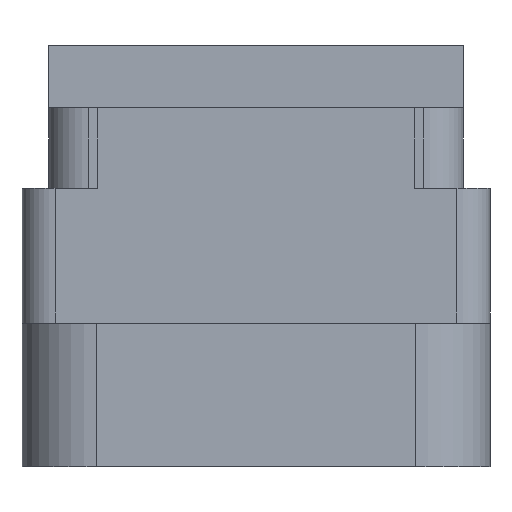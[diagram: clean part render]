
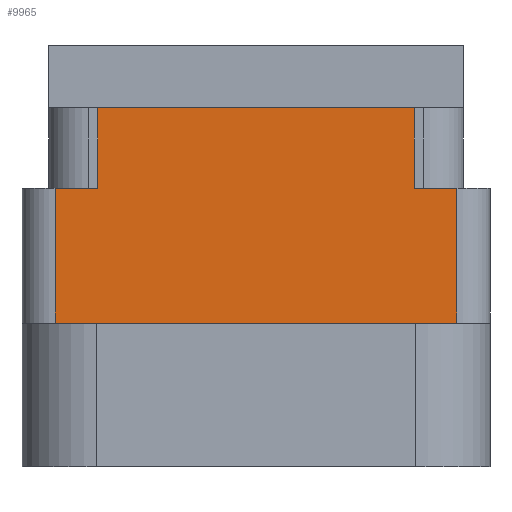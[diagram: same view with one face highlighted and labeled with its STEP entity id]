
A CAD part, left-side view. The second image highlights one B-rep face of the part: STEP entity #9965.
In plain terms, the highlighted planar face has unit normal (-1, 0, 0).
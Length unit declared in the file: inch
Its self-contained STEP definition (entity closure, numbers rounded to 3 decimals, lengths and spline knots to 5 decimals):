
#781 = ORIENTED_EDGE ( 'NONE', *, *, #7627, .F. ) ;
#800 = DIRECTION ( 'NONE',  ( 0., 0., -1. ) ) ;
#829 = CARTESIAN_POINT ( 'NONE',  ( -1., 0., -0.52 ) ) ;
#1359 = CARTESIAN_POINT ( 'NONE',  ( -1., 0.438, -0.117 ) ) ;
#2699 = ORIENTED_EDGE ( 'NONE', *, *, #14795, .T. ) ;
#3583 = LINE ( 'NONE', #25092, #16459 ) ;
#4139 = PLANE ( 'NONE',  #21586 ) ;
#4906 = LINE ( 'NONE', #26432, #11328 ) ;
#5206 = CARTESIAN_POINT ( 'NONE',  ( -1., -0.296, -0.268 ) ) ;
#5990 = ORIENTED_EDGE ( 'NONE', *, *, #13882, .F. ) ;
#6275 = VECTOR ( 'NONE', #800, 39.37008 ) ;
#7132 = VECTOR ( 'NONE', #29669, 39.37008 ) ;
#7178 = VERTEX_POINT ( 'NONE', #7757 ) ;
#7310 = CARTESIAN_POINT ( 'NONE',  ( -1., 0.376, -0.789 ) ) ;
#7619 = CARTESIAN_POINT ( 'NONE',  ( -1., 0.296, -0.268 ) ) ;
#7627 = EDGE_CURVE ( 'NONE', #20608, #7178, #20524, .T. ) ;
#7757 = CARTESIAN_POINT ( 'NONE',  ( -1., 0.296, -0.117 ) ) ;
#8658 = CARTESIAN_POINT ( 'NONE',  ( -1., -0.438, -0.789 ) ) ;
#8697 = CARTESIAN_POINT ( 'NONE',  ( -1., 0.376, -0.268 ) ) ;
#9180 = CARTESIAN_POINT ( 'NONE',  ( -1., -0.376, -0.789 ) ) ;
#9965 = ADVANCED_FACE ( 'NONE', ( #15332 ), #4139, .T. ) ;
#10015 = DIRECTION ( 'NONE',  ( 0., 0., 1. ) ) ;
#10758 = ORIENTED_EDGE ( 'NONE', *, *, #21530, .T. ) ;
#11161 = LINE ( 'NONE', #829, #17992 ) ;
#11328 = VECTOR ( 'NONE', #20034, 39.37008 ) ;
#12060 = EDGE_LOOP ( 'NONE', ( #5990, #2699, #23293, #23533, #17373, #10758, #25731, #781 ) ) ;
#12412 = VERTEX_POINT ( 'NONE', #27293 ) ;
#13398 = EDGE_CURVE ( 'NONE', #14113, #15304, #16719, .T. ) ;
#13882 = EDGE_CURVE ( 'NONE', #17393, #20608, #4906, .T. ) ;
#14113 = VERTEX_POINT ( 'NONE', #5206 ) ;
#14179 = CARTESIAN_POINT ( 'NONE',  ( -1., -0.376, -0.268 ) ) ;
#14795 = EDGE_CURVE ( 'NONE', #17393, #21292, #26772, .T. ) ;
#15304 = VERTEX_POINT ( 'NONE', #14179 ) ;
#15332 = FACE_OUTER_BOUND ( 'NONE', #12060, .T. ) ;
#15593 = EDGE_CURVE ( 'NONE', #7178, #12412, #18391, .T. ) ;
#15826 = DIRECTION ( 'NONE',  ( 0., 0., 1. ) ) ;
#16459 = VECTOR ( 'NONE', #27239, 39.37008 ) ;
#16564 = CARTESIAN_POINT ( 'NONE',  ( -1., 0.296, -0.268 ) ) ;
#16719 = LINE ( 'NONE', #17716, #18182 ) ;
#16848 = EDGE_CURVE ( 'NONE', #21292, #17653, #11161, .T. ) ;
#17303 = VECTOR ( 'NONE', #10015, 39.37008 ) ;
#17372 = DIRECTION ( 'NONE',  ( 0., -1., 0. ) ) ;
#17373 = ORIENTED_EDGE ( 'NONE', *, *, #13398, .F. ) ;
#17393 = VERTEX_POINT ( 'NONE', #8697 ) ;
#17653 = VERTEX_POINT ( 'NONE', #21670 ) ;
#17716 = CARTESIAN_POINT ( 'NONE',  ( -1., 0., -0.268 ) ) ;
#17992 = VECTOR ( 'NONE', #19053, 39.37008 ) ;
#18182 = VECTOR ( 'NONE', #24490, 39.37008 ) ;
#18391 = LINE ( 'NONE', #1359, #25974 ) ;
#19053 = DIRECTION ( 'NONE',  ( 0., -1., 0. ) ) ;
#20034 = DIRECTION ( 'NONE',  ( 0., -1., 0. ) ) ;
#20058 = DIRECTION ( 'NONE',  ( -1., 0., 0. ) ) ;
#20524 = LINE ( 'NONE', #7619, #17303 ) ;
#20608 = VERTEX_POINT ( 'NONE', #16564 ) ;
#21292 = VERTEX_POINT ( 'NONE', #25923 ) ;
#21530 = EDGE_CURVE ( 'NONE', #14113, #12412, #3583, .T. ) ;
#21586 = AXIS2_PLACEMENT_3D ( 'NONE', #8658, #20058, #15826 ) ;
#21670 = CARTESIAN_POINT ( 'NONE',  ( -1., -0.376, -0.52 ) ) ;
#23293 = ORIENTED_EDGE ( 'NONE', *, *, #16848, .T. ) ;
#23533 = ORIENTED_EDGE ( 'NONE', *, *, #24955, .T. ) ;
#24490 = DIRECTION ( 'NONE',  ( 0., -1., 0. ) ) ;
#24955 = EDGE_CURVE ( 'NONE', #17653, #15304, #27646, .T. ) ;
#25092 = CARTESIAN_POINT ( 'NONE',  ( -1., -0.296, -0.268 ) ) ;
#25731 = ORIENTED_EDGE ( 'NONE', *, *, #15593, .F. ) ;
#25923 = CARTESIAN_POINT ( 'NONE',  ( -1., 0.376, -0.52 ) ) ;
#25974 = VECTOR ( 'NONE', #17372, 39.37008 ) ;
#26432 = CARTESIAN_POINT ( 'NONE',  ( -1., 0., -0.268 ) ) ;
#26772 = LINE ( 'NONE', #7310, #6275 ) ;
#27239 = DIRECTION ( 'NONE',  ( 0., 0., 1. ) ) ;
#27293 = CARTESIAN_POINT ( 'NONE',  ( -1., -0.296, -0.117 ) ) ;
#27646 = LINE ( 'NONE', #9180, #7132 ) ;
#29669 = DIRECTION ( 'NONE',  ( 0., 0., 1. ) ) ;
